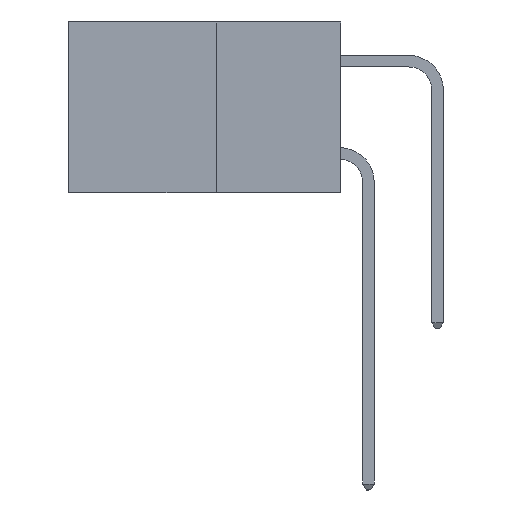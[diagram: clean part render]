
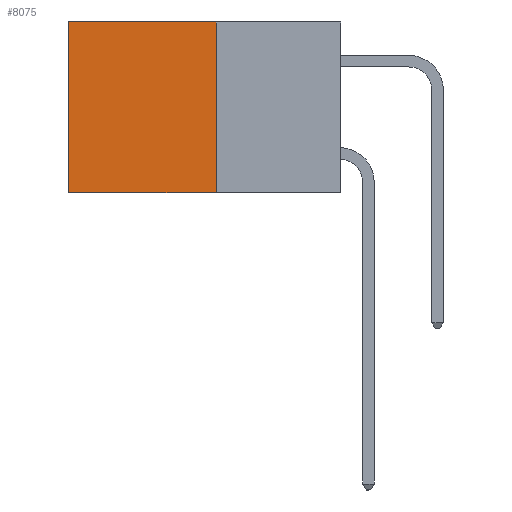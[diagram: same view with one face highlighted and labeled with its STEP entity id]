
A CAD part, left-side view. The second image highlights one B-rep face of the part: STEP entity #8075.
In plain terms, the highlighted planar face has unit normal (-1, 0, 0).
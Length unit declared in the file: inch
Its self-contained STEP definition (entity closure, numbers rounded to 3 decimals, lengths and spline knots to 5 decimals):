
#209 = EDGE_CURVE ( 'NONE', #7224, #6663, #2847, .T. ) ;
#296 = CARTESIAN_POINT ( 'NONE',  ( 0.277, 0.59, -0.37 ) ) ;
#450 = ORIENTED_EDGE ( 'NONE', *, *, #6583, .F. ) ;
#524 = DIRECTION ( 'NONE',  ( 0., 0., -1. ) ) ;
#683 = CARTESIAN_POINT ( 'NONE',  ( 0.277, 0.27, 0. ) ) ;
#875 = VERTEX_POINT ( 'NONE', #9488 ) ;
#1571 = LINE ( 'NONE', #8609, #3308 ) ;
#1716 = DIRECTION ( 'NONE',  ( 0., 1., 0. ) ) ;
#2214 = VECTOR ( 'NONE', #1716, 39.37008 ) ;
#2322 = CARTESIAN_POINT ( 'NONE',  ( 0.277, 0.27, -0.37 ) ) ;
#2429 = PLANE ( 'NONE',  #6333 ) ;
#2566 = CARTESIAN_POINT ( 'NONE',  ( 0.277, 0.27, 0. ) ) ;
#2847 = LINE ( 'NONE', #2322, #4029 ) ;
#2949 = LINE ( 'NONE', #2566, #9242 ) ;
#3060 = DIRECTION ( 'NONE',  ( 0., 1., 0. ) ) ;
#3292 = DIRECTION ( 'NONE',  ( 0., 0., -1. ) ) ;
#3308 = VECTOR ( 'NONE', #524, 39.37008 ) ;
#3574 = ORIENTED_EDGE ( 'NONE', *, *, #5529, .T. ) ;
#3980 = EDGE_CURVE ( 'NONE', #7224, #875, #2949, .T. ) ;
#4029 = VECTOR ( 'NONE', #9558, 39.37008 ) ;
#4356 = ORIENTED_EDGE ( 'NONE', *, *, #209, .F. ) ;
#4374 = FACE_OUTER_BOUND ( 'NONE', #8399, .T. ) ;
#4451 = LINE ( 'NONE', #8844, #2214 ) ;
#5529 = EDGE_CURVE ( 'NONE', #875, #9596, #1571, .T. ) ;
#6333 = AXIS2_PLACEMENT_3D ( 'NONE', #9003, #8232, #3292 ) ;
#6583 = EDGE_CURVE ( 'NONE', #6663, #9596, #4451, .T. ) ;
#6663 = VERTEX_POINT ( 'NONE', #8461 ) ;
#7104 = ORIENTED_EDGE ( 'NONE', *, *, #3980, .T. ) ;
#7224 = VERTEX_POINT ( 'NONE', #683 ) ;
#8075 = ADVANCED_FACE ( 'NONE', ( #4374 ), #2429, .F. ) ;
#8232 = DIRECTION ( 'NONE',  ( 1., 0., 0. ) ) ;
#8399 = EDGE_LOOP ( 'NONE', ( #3574, #450, #4356, #7104 ) ) ;
#8461 = CARTESIAN_POINT ( 'NONE',  ( 0.277, 0.27, -0.37 ) ) ;
#8609 = CARTESIAN_POINT ( 'NONE',  ( 0.277, 0.59, -0.37 ) ) ;
#8844 = CARTESIAN_POINT ( 'NONE',  ( 0.277, 0.27, -0.37 ) ) ;
#9003 = CARTESIAN_POINT ( 'NONE',  ( 0.277, 0.27, -0.37 ) ) ;
#9242 = VECTOR ( 'NONE', #3060, 39.37008 ) ;
#9488 = CARTESIAN_POINT ( 'NONE',  ( 0.277, 0.59, 0. ) ) ;
#9558 = DIRECTION ( 'NONE',  ( 0., 0., -1. ) ) ;
#9596 = VERTEX_POINT ( 'NONE', #296 ) ;
